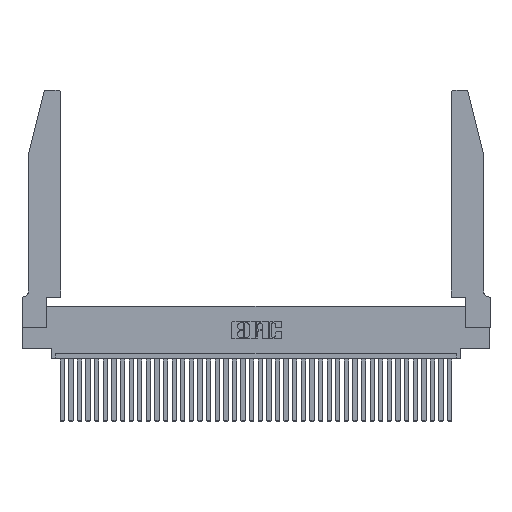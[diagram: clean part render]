
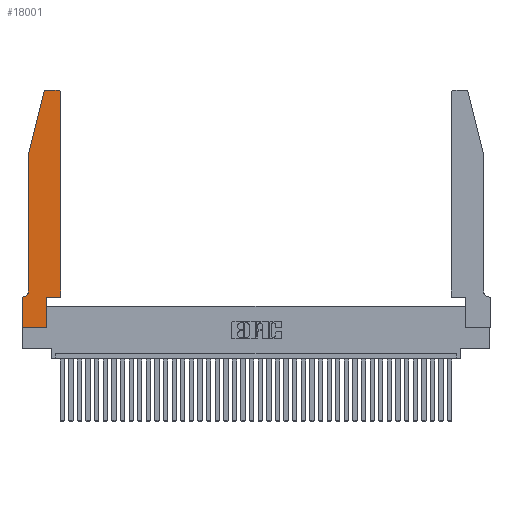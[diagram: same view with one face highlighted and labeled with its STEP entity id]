
A CAD part, top view. The second image highlights one B-rep face of the part: STEP entity #18001.
In plain terms, the highlighted planar face has unit normal (0, 0, 1).
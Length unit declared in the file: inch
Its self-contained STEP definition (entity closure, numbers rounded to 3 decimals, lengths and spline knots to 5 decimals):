
#491 = CARTESIAN_POINT ( 'NONE',  ( 0., 0.35, 0.37 ) ) ;
#854 = EDGE_CURVE ( 'NONE', #21065, #30573, #12315, .T. ) ;
#1199 = EDGE_CURVE ( 'NONE', #28102, #34339, #28259, .T. ) ;
#1354 = VECTOR ( 'NONE', #35793, 39.37008 ) ;
#1818 = AXIS2_PLACEMENT_3D ( 'NONE', #3130, #30110, #12147 ) ;
#2342 = ORIENTED_EDGE ( 'NONE', *, *, #31262, .T. ) ;
#3130 = CARTESIAN_POINT ( 'NONE',  ( 0.4205, 2.72, 0.37 ) ) ;
#3980 = CARTESIAN_POINT ( 'NONE',  ( 0.4505, 0.35, 0.37 ) ) ;
#4181 = EDGE_CURVE ( 'NONE', #33804, #18172, #8030, .T. ) ;
#4245 = FACE_OUTER_BOUND ( 'NONE', #30536, .T. ) ;
#4683 = LINE ( 'NONE', #19407, #17341 ) ;
#5007 = DIRECTION ( 'NONE',  ( 0., 0., -1. ) ) ;
#5967 = LINE ( 'NONE', #31381, #28435 ) ;
#6261 = ORIENTED_EDGE ( 'NONE', *, *, #1199, .T. ) ;
#6899 = CARTESIAN_POINT ( 'NONE',  ( 0., 0., 0.37 ) ) ;
#6919 = DIRECTION ( 'NONE',  ( -1., 0., 0. ) ) ;
#7983 = EDGE_CURVE ( 'NONE', #26613, #28102, #15202, .T. ) ;
#8030 = LINE ( 'NONE', #18211, #22058 ) ;
#8164 = ORIENTED_EDGE ( 'NONE', *, *, #10538, .T. ) ;
#8269 = VERTEX_POINT ( 'NONE', #28576 ) ;
#9048 = DIRECTION ( 'NONE',  ( 0., 1., 0. ) ) ;
#9081 = CARTESIAN_POINT ( 'NONE',  ( 0.4205, 2.75, 0.37 ) ) ;
#9652 = LINE ( 'NONE', #10743, #26115 ) ;
#10538 = EDGE_CURVE ( 'NONE', #8269, #21065, #26803, .T. ) ;
#10743 = CARTESIAN_POINT ( 'NONE',  ( 0., 0., 0.37 ) ) ;
#10939 = DIRECTION ( 'NONE',  ( 1., 0., 0. ) ) ;
#11284 = DIRECTION ( 'NONE',  ( -1., 0., 0. ) ) ;
#11640 = CARTESIAN_POINT ( 'NONE',  ( 0., 0.35, 0.37 ) ) ;
#11942 = EDGE_CURVE ( 'NONE', #14946, #33556, #4683, .T. ) ;
#12000 = VERTEX_POINT ( 'NONE', #37285 ) ;
#12147 = DIRECTION ( 'NONE',  ( 1., 0., 0. ) ) ;
#12199 = ORIENTED_EDGE ( 'NONE', *, *, #7983, .T. ) ;
#12315 = CIRCLE ( 'NONE', #1818, 0.03 ) ;
#12387 = CARTESIAN_POINT ( 'NONE',  ( 0.2865, 0.35, 0.37 ) ) ;
#12533 = CARTESIAN_POINT ( 'NONE',  ( 0.284, 2.75, 0.37 ) ) ;
#12553 = CIRCLE ( 'NONE', #24724, 0.03 ) ;
#12875 = DIRECTION ( 'NONE',  ( 1., 0., 0. ) ) ;
#13310 = DIRECTION ( 'NONE',  ( 1., 0., 0. ) ) ;
#13852 = CARTESIAN_POINT ( 'NONE',  ( 0.4505, 2.72, 0.37 ) ) ;
#14170 = CARTESIAN_POINT ( 'NONE',  ( 0.0755, 2., 0.37 ) ) ;
#14373 = ORIENTED_EDGE ( 'NONE', *, *, #31236, .T. ) ;
#14946 = VERTEX_POINT ( 'NONE', #21547 ) ;
#15202 = CIRCLE ( 'NONE', #37808, 0.07 ) ;
#15618 = CARTESIAN_POINT ( 'NONE',  ( 0.0055, 0.42, 0.37 ) ) ;
#15888 = DIRECTION ( 'NONE',  ( 0., 0., 1. ) ) ;
#15938 = PLANE ( 'NONE',  #29028 ) ;
#16038 = DIRECTION ( 'NONE',  ( 0., -1., 0. ) ) ;
#16488 = DIRECTION ( 'NONE',  ( 0., -1., 0. ) ) ;
#16634 = EDGE_CURVE ( 'NONE', #18172, #8269, #32938, .T. ) ;
#17341 = VECTOR ( 'NONE', #34020, 39.37008 ) ;
#17721 = VERTEX_POINT ( 'NONE', #12533 ) ;
#17875 = VECTOR ( 'NONE', #28036, 39.37008 ) ;
#18001 = ADVANCED_FACE ( 'NONE', ( #4245 ), #15938, .T. ) ;
#18172 = VERTEX_POINT ( 'NONE', #12387 ) ;
#18211 = CARTESIAN_POINT ( 'NONE',  ( 0.2865, 0.35, 0.37 ) ) ;
#18243 = ORIENTED_EDGE ( 'NONE', *, *, #4181, .T. ) ;
#19407 = CARTESIAN_POINT ( 'NONE',  ( 0.0755, 2., 0.37 ) ) ;
#19721 = CARTESIAN_POINT ( 'NONE',  ( 0.0055, 0.35, 0.37 ) ) ;
#20562 = EDGE_CURVE ( 'NONE', #34339, #12000, #9652, .T. ) ;
#20873 = CARTESIAN_POINT ( 'NONE',  ( 0.2865, 0., 0.37 ) ) ;
#20985 = LINE ( 'NONE', #27979, #38280 ) ;
#21065 = VERTEX_POINT ( 'NONE', #13852 ) ;
#21547 = CARTESIAN_POINT ( 'NONE',  ( 0.25487, 2.72718, 0.37 ) ) ;
#22058 = VECTOR ( 'NONE', #9048, 39.37008 ) ;
#23140 = VECTOR ( 'NONE', #10939, 39.37008 ) ;
#24380 = EDGE_CURVE ( 'NONE', #33556, #26613, #20985, .T. ) ;
#24724 = AXIS2_PLACEMENT_3D ( 'NONE', #24820, #15888, #12875 ) ;
#24820 = CARTESIAN_POINT ( 'NONE',  ( 0.284, 2.72, 0.37 ) ) ;
#26115 = VECTOR ( 'NONE', #16488, 39.37008 ) ;
#26613 = VERTEX_POINT ( 'NONE', #29311 ) ;
#26704 = LINE ( 'NONE', #6899, #1354 ) ;
#26803 = LINE ( 'NONE', #28175, #17875 ) ;
#26846 = ORIENTED_EDGE ( 'NONE', *, *, #11942, .T. ) ;
#27568 = ORIENTED_EDGE ( 'NONE', *, *, #24380, .T. ) ;
#27979 = CARTESIAN_POINT ( 'NONE',  ( 0.0755, 2., 0.37 ) ) ;
#28036 = DIRECTION ( 'NONE',  ( 0., 1., 0. ) ) ;
#28102 = VERTEX_POINT ( 'NONE', #19721 ) ;
#28153 = DIRECTION ( 'NONE',  ( 0., 0., 1. ) ) ;
#28175 = CARTESIAN_POINT ( 'NONE',  ( 0.4505, 0.35, 0.37 ) ) ;
#28238 = ORIENTED_EDGE ( 'NONE', *, *, #20562, .T. ) ;
#28259 = LINE ( 'NONE', #28798, #33862 ) ;
#28435 = VECTOR ( 'NONE', #6919, 39.37008 ) ;
#28576 = CARTESIAN_POINT ( 'NONE',  ( 0.4505, 0.35, 0.37 ) ) ;
#28798 = CARTESIAN_POINT ( 'NONE',  ( 0.0755, 0.35, 0.37 ) ) ;
#29028 = AXIS2_PLACEMENT_3D ( 'NONE', #491, #28153, #13310 ) ;
#29311 = CARTESIAN_POINT ( 'NONE',  ( 0.0755, 0.42, 0.37 ) ) ;
#29349 = EDGE_CURVE ( 'NONE', #30573, #17721, #5967, .T. ) ;
#30110 = DIRECTION ( 'NONE',  ( 0., 0., 1. ) ) ;
#30536 = EDGE_LOOP ( 'NONE', ( #34593, #14373, #26846, #27568, #12199, #6261, #28238, #2342, #18243, #32694, #8164, #33711 ) ) ;
#30573 = VERTEX_POINT ( 'NONE', #9081 ) ;
#31236 = EDGE_CURVE ( 'NONE', #17721, #14946, #12553, .T. ) ;
#31262 = EDGE_CURVE ( 'NONE', #12000, #33804, #26704, .T. ) ;
#31381 = CARTESIAN_POINT ( 'NONE',  ( 0.2605, 2.75, 0.37 ) ) ;
#31918 = DIRECTION ( 'NONE',  ( -1., 0., 0. ) ) ;
#32694 = ORIENTED_EDGE ( 'NONE', *, *, #16634, .T. ) ;
#32938 = LINE ( 'NONE', #3980, #23140 ) ;
#33556 = VERTEX_POINT ( 'NONE', #14170 ) ;
#33711 = ORIENTED_EDGE ( 'NONE', *, *, #854, .T. ) ;
#33804 = VERTEX_POINT ( 'NONE', #20873 ) ;
#33862 = VECTOR ( 'NONE', #31918, 39.37008 ) ;
#34020 = DIRECTION ( 'NONE',  ( -0.239, -0.971, 0. ) ) ;
#34339 = VERTEX_POINT ( 'NONE', #11640 ) ;
#34593 = ORIENTED_EDGE ( 'NONE', *, *, #29349, .T. ) ;
#35793 = DIRECTION ( 'NONE',  ( 1., 0., 0. ) ) ;
#37285 = CARTESIAN_POINT ( 'NONE',  ( 0., 0., 0.37 ) ) ;
#37808 = AXIS2_PLACEMENT_3D ( 'NONE', #15618, #5007, #11284 ) ;
#38280 = VECTOR ( 'NONE', #16038, 39.37008 ) ;
